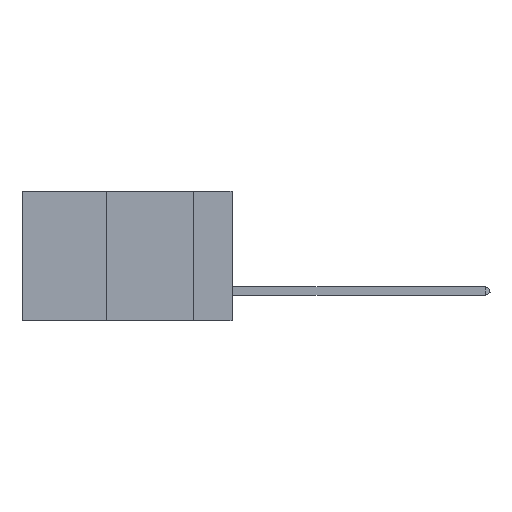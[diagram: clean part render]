
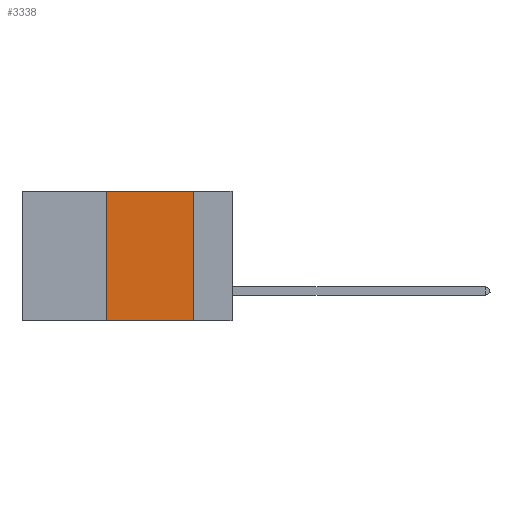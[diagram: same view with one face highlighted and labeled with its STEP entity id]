
A CAD part, left-side view. The second image highlights one B-rep face of the part: STEP entity #3338.
In plain terms, the highlighted planar face has unit normal (-1, 0, 0).
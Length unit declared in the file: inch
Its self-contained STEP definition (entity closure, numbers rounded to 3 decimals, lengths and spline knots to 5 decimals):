
#1453 = DIRECTION ( 'NONE',  ( 0., -1., 0. ) ) ;
#2373 = CARTESIAN_POINT ( 'NONE',  ( 0., 0.6, 0. ) ) ;
#2550 = DIRECTION ( 'NONE',  ( 1., 0., 0. ) ) ;
#2902 = PLANE ( 'NONE',  #20286 ) ;
#3338 = ADVANCED_FACE ( 'NONE', ( #3496 ), #2902, .F. ) ;
#3496 = FACE_OUTER_BOUND ( 'NONE', #47098, .T. ) ;
#3530 = LINE ( 'NONE', #6653, #38097 ) ;
#3788 = VERTEX_POINT ( 'NONE', #20512 ) ;
#6484 = CARTESIAN_POINT ( 'NONE',  ( 0., 0.36, 0. ) ) ;
#6499 = DIRECTION ( 'NONE',  ( 0., 0., -1. ) ) ;
#6653 = CARTESIAN_POINT ( 'NONE',  ( 0., 0.11, 0. ) ) ;
#10512 = VECTOR ( 'NONE', #1453, 39.37008 ) ;
#11101 = LINE ( 'NONE', #13635, #10512 ) ;
#11411 = LINE ( 'NONE', #44475, #19927 ) ;
#12904 = VECTOR ( 'NONE', #22238, 39.37008 ) ;
#13635 = CARTESIAN_POINT ( 'NONE',  ( 0., 0.6, -0.37 ) ) ;
#14835 = ORIENTED_EDGE ( 'NONE', *, *, #17888, .F. ) ;
#16883 = VERTEX_POINT ( 'NONE', #22579 ) ;
#17888 = EDGE_CURVE ( 'NONE', #16883, #36304, #11411, .T. ) ;
#19927 = VECTOR ( 'NONE', #44128, 39.37008 ) ;
#20286 = AXIS2_PLACEMENT_3D ( 'NONE', #2373, #2550, #6499 ) ;
#20512 = CARTESIAN_POINT ( 'NONE',  ( 0., 0.11, -0.37 ) ) ;
#22238 = DIRECTION ( 'NONE',  ( 0., 0., 1. ) ) ;
#22579 = CARTESIAN_POINT ( 'NONE',  ( 0., 0.36, 0. ) ) ;
#22594 = ORIENTED_EDGE ( 'NONE', *, *, #26366, .T. ) ;
#26105 = DIRECTION ( 'NONE',  ( 0., 0., -1. ) ) ;
#26366 = EDGE_CURVE ( 'NONE', #40410, #3788, #11101, .T. ) ;
#29751 = ORIENTED_EDGE ( 'NONE', *, *, #40709, .F. ) ;
#31416 = CARTESIAN_POINT ( 'NONE',  ( 0., 0.11, 0. ) ) ;
#36304 = VERTEX_POINT ( 'NONE', #31416 ) ;
#36448 = CARTESIAN_POINT ( 'NONE',  ( 0., 0.36, -0.37 ) ) ;
#38097 = VECTOR ( 'NONE', #26105, 39.37008 ) ;
#38685 = EDGE_CURVE ( 'NONE', #40410, #16883, #47461, .T. ) ;
#40410 = VERTEX_POINT ( 'NONE', #36448 ) ;
#40709 = EDGE_CURVE ( 'NONE', #36304, #3788, #3530, .T. ) ;
#44128 = DIRECTION ( 'NONE',  ( 0., -1., 0. ) ) ;
#44475 = CARTESIAN_POINT ( 'NONE',  ( 0., 0.6, 0. ) ) ;
#45974 = ORIENTED_EDGE ( 'NONE', *, *, #38685, .F. ) ;
#47098 = EDGE_LOOP ( 'NONE', ( #29751, #14835, #45974, #22594 ) ) ;
#47461 = LINE ( 'NONE', #6484, #12904 ) ;
